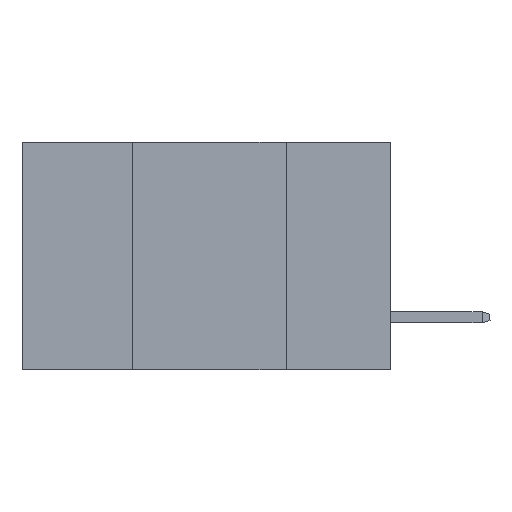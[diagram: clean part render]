
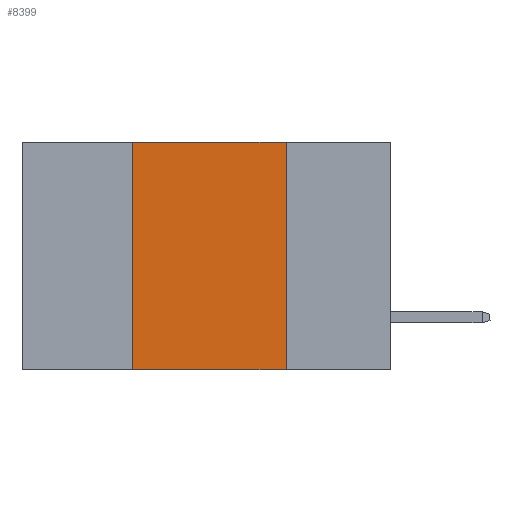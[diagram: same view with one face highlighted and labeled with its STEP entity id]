
A CAD part, left-side view. The second image highlights one B-rep face of the part: STEP entity #8399.
In plain terms, the highlighted planar face has unit normal (-1, 0, 0).
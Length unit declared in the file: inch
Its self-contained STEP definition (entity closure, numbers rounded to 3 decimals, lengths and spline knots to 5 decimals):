
#67 = ORIENTED_EDGE ( 'NONE', *, *, #7393, .T. ) ;
#170 = EDGE_LOOP ( 'NONE', ( #4544, #12111, #4865, #67 ) ) ;
#509 = EDGE_CURVE ( 'NONE', #8393, #1112, #9935, .T. ) ;
#852 = DIRECTION ( 'NONE',  ( 0., -1., 0. ) ) ;
#853 = CARTESIAN_POINT ( 'NONE',  ( 0., 0.17, -0.37 ) ) ;
#874 = VERTEX_POINT ( 'NONE', #5282 ) ;
#1086 = CARTESIAN_POINT ( 'NONE',  ( 0., 0.17, 0. ) ) ;
#1112 = VERTEX_POINT ( 'NONE', #853 ) ;
#1829 = VECTOR ( 'NONE', #8375, 39.37008 ) ;
#2156 = PLANE ( 'NONE',  #2736 ) ;
#2284 = FACE_OUTER_BOUND ( 'NONE', #170, .T. ) ;
#2736 = AXIS2_PLACEMENT_3D ( 'NONE', #10739, #8866, #3130 ) ;
#3025 = CARTESIAN_POINT ( 'NONE',  ( 0., 0.17, 0. ) ) ;
#3130 = DIRECTION ( 'NONE',  ( 0., 0., -1. ) ) ;
#3858 = CARTESIAN_POINT ( 'NONE',  ( 0., 0.42, 0. ) ) ;
#4448 = LINE ( 'NONE', #12142, #1829 ) ;
#4544 = ORIENTED_EDGE ( 'NONE', *, *, #509, .F. ) ;
#4865 = ORIENTED_EDGE ( 'NONE', *, *, #11201, .F. ) ;
#4910 = LINE ( 'NONE', #12431, #9650 ) ;
#5282 = CARTESIAN_POINT ( 'NONE',  ( 0., 0.42, -0.37 ) ) ;
#5550 = CARTESIAN_POINT ( 'NONE',  ( 0., 0.42, 0. ) ) ;
#7393 = EDGE_CURVE ( 'NONE', #874, #1112, #4448, .T. ) ;
#7414 = VECTOR ( 'NONE', #11690, 39.37008 ) ;
#7575 = EDGE_CURVE ( 'NONE', #12185, #8393, #4910, .T. ) ;
#8375 = DIRECTION ( 'NONE',  ( 0., -1., 0. ) ) ;
#8393 = VERTEX_POINT ( 'NONE', #1086 ) ;
#8399 = ADVANCED_FACE ( 'NONE', ( #2284 ), #2156, .F. ) ;
#8866 = DIRECTION ( 'NONE',  ( 1., 0., 0. ) ) ;
#8962 = VECTOR ( 'NONE', #10510, 39.37008 ) ;
#9262 = LINE ( 'NONE', #3858, #8962 ) ;
#9650 = VECTOR ( 'NONE', #852, 39.37008 ) ;
#9935 = LINE ( 'NONE', #3025, #7414 ) ;
#10510 = DIRECTION ( 'NONE',  ( 0., 0., 1. ) ) ;
#10739 = CARTESIAN_POINT ( 'NONE',  ( 0., 0.6, 0. ) ) ;
#11201 = EDGE_CURVE ( 'NONE', #874, #12185, #9262, .T. ) ;
#11690 = DIRECTION ( 'NONE',  ( 0., 0., -1. ) ) ;
#12111 = ORIENTED_EDGE ( 'NONE', *, *, #7575, .F. ) ;
#12142 = CARTESIAN_POINT ( 'NONE',  ( 0., 0.6, -0.37 ) ) ;
#12185 = VERTEX_POINT ( 'NONE', #5550 ) ;
#12431 = CARTESIAN_POINT ( 'NONE',  ( 0., 0.6, 0. ) ) ;
